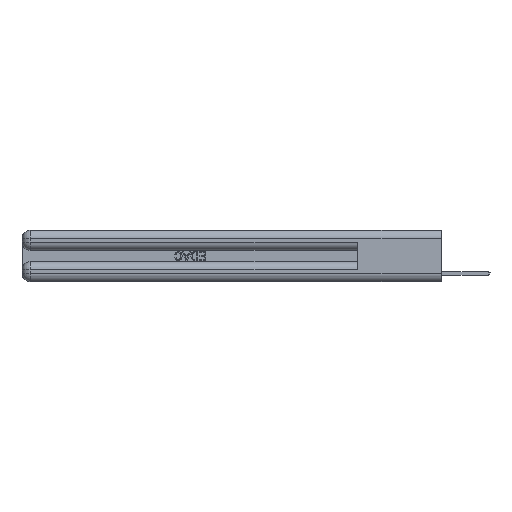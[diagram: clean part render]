
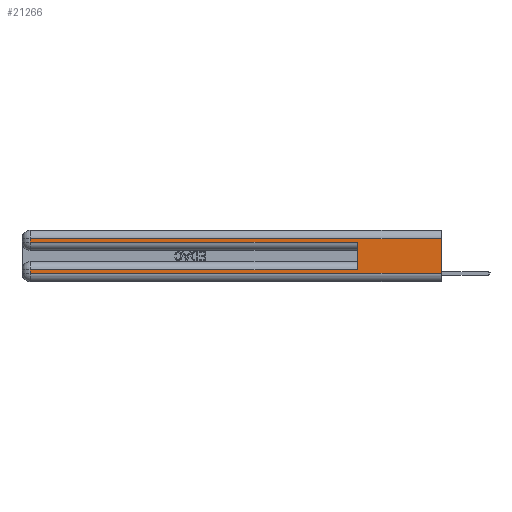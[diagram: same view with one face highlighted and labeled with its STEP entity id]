
A CAD part, left-side view. The second image highlights one B-rep face of the part: STEP entity #21266.
In plain terms, the highlighted planar face has unit normal (-1, 0, 0).
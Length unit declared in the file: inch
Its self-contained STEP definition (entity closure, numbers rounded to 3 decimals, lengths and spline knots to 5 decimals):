
#546 = DIRECTION ( 'NONE',  ( 1., 0., 0. ) ) ;
#887 = LINE ( 'NONE', #25383, #1001 ) ;
#1001 = VECTOR ( 'NONE', #10462, 39.37008 ) ;
#1051 = VECTOR ( 'NONE', #24910, 39.37008 ) ;
#1448 = AXIS2_PLACEMENT_3D ( 'NONE', #28660, #546, #10932 ) ;
#1958 = CARTESIAN_POINT ( 'NONE',  ( 0., 2.94, 0.06 ) ) ;
#3418 = CARTESIAN_POINT ( 'NONE',  ( 0., 0., 0.31 ) ) ;
#3622 = CARTESIAN_POINT ( 'NONE',  ( 0., 0.6, 0.085 ) ) ;
#4001 = DIRECTION ( 'NONE',  ( 0., -1., 0. ) ) ;
#4918 = VERTEX_POINT ( 'NONE', #3418 ) ;
#4954 = CARTESIAN_POINT ( 'NONE',  ( 0., 2.94, 0.31 ) ) ;
#4985 = CARTESIAN_POINT ( 'NONE',  ( 0., 2.94, 0.285 ) ) ;
#5174 = VERTEX_POINT ( 'NONE', #1958 ) ;
#5226 = EDGE_CURVE ( 'NONE', #13327, #26581, #20257, .T. ) ;
#5734 = LINE ( 'NONE', #5896, #10826 ) ;
#5896 = CARTESIAN_POINT ( 'NONE',  ( 0., 2.94, 0.37 ) ) ;
#7226 = ORIENTED_EDGE ( 'NONE', *, *, #17500, .T. ) ;
#7757 = VERTEX_POINT ( 'NONE', #12600 ) ;
#8492 = CARTESIAN_POINT ( 'NONE',  ( 0., 0.6, 0.285 ) ) ;
#9672 = LINE ( 'NONE', #22571, #1051 ) ;
#9835 = LINE ( 'NONE', #30186, #29101 ) ;
#9918 = VERTEX_POINT ( 'NONE', #8492 ) ;
#10306 = EDGE_CURVE ( 'NONE', #4918, #7757, #30637, .T. ) ;
#10462 = DIRECTION ( 'NONE',  ( 0., 0., 1. ) ) ;
#10665 = VECTOR ( 'NONE', #4001, 39.37008 ) ;
#10826 = VECTOR ( 'NONE', #20621, 39.37008 ) ;
#10932 = DIRECTION ( 'NONE',  ( 0., 0., -1. ) ) ;
#11837 = EDGE_CURVE ( 'NONE', #5174, #7757, #24356, .T. ) ;
#12512 = VECTOR ( 'NONE', #26177, 39.37008 ) ;
#12564 = ORIENTED_EDGE ( 'NONE', *, *, #10306, .F. ) ;
#12600 = CARTESIAN_POINT ( 'NONE',  ( 0., 0., 0.06 ) ) ;
#12888 = ORIENTED_EDGE ( 'NONE', *, *, #11837, .T. ) ;
#13202 = ORIENTED_EDGE ( 'NONE', *, *, #5226, .T. ) ;
#13327 = VERTEX_POINT ( 'NONE', #3622 ) ;
#13931 = EDGE_LOOP ( 'NONE', ( #12564, #22596, #7226, #15927, #15708, #13202, #24129, #12888 ) ) ;
#13957 = VECTOR ( 'NONE', #14703, 39.37008 ) ;
#14703 = DIRECTION ( 'NONE',  ( 0., -1., 0. ) ) ;
#15708 = ORIENTED_EDGE ( 'NONE', *, *, #23524, .F. ) ;
#15927 = ORIENTED_EDGE ( 'NONE', *, *, #18769, .T. ) ;
#16229 = CARTESIAN_POINT ( 'NONE',  ( 0., 0., 0.37 ) ) ;
#16570 = CARTESIAN_POINT ( 'NONE',  ( 0., 0., 0.06 ) ) ;
#17500 = EDGE_CURVE ( 'NONE', #18907, #27612, #5734, .T. ) ;
#18769 = EDGE_CURVE ( 'NONE', #27612, #9918, #22007, .T. ) ;
#18907 = VERTEX_POINT ( 'NONE', #4954 ) ;
#19912 = DIRECTION ( 'NONE',  ( 0., 1., 0. ) ) ;
#20200 = VECTOR ( 'NONE', #30690, 39.37008 ) ;
#20257 = LINE ( 'NONE', #27588, #20200 ) ;
#20621 = DIRECTION ( 'NONE',  ( 0., 0., -1. ) ) ;
#21266 = ADVANCED_FACE ( 'NONE', ( #31299 ), #25684, .F. ) ;
#22007 = LINE ( 'NONE', #32107, #13957 ) ;
#22571 = CARTESIAN_POINT ( 'NONE',  ( 0., 2.94, 0.37 ) ) ;
#22596 = ORIENTED_EDGE ( 'NONE', *, *, #27273, .T. ) ;
#23524 = EDGE_CURVE ( 'NONE', #13327, #9918, #887, .T. ) ;
#24129 = ORIENTED_EDGE ( 'NONE', *, *, #26157, .T. ) ;
#24356 = LINE ( 'NONE', #16570, #10665 ) ;
#24821 = CARTESIAN_POINT ( 'NONE',  ( 0., 2.94, 0.085 ) ) ;
#24910 = DIRECTION ( 'NONE',  ( 0., 0., -1. ) ) ;
#25383 = CARTESIAN_POINT ( 'NONE',  ( 0., 0.6, 0.145 ) ) ;
#25684 = PLANE ( 'NONE',  #1448 ) ;
#26157 = EDGE_CURVE ( 'NONE', #26581, #5174, #9672, .T. ) ;
#26177 = DIRECTION ( 'NONE',  ( 0., 0., -1. ) ) ;
#26581 = VERTEX_POINT ( 'NONE', #24821 ) ;
#27273 = EDGE_CURVE ( 'NONE', #4918, #18907, #9835, .T. ) ;
#27588 = CARTESIAN_POINT ( 'NONE',  ( 0., 0., 0.085 ) ) ;
#27612 = VERTEX_POINT ( 'NONE', #4985 ) ;
#28660 = CARTESIAN_POINT ( 'NONE',  ( 0., 0., 0.37 ) ) ;
#29101 = VECTOR ( 'NONE', #19912, 39.37008 ) ;
#30186 = CARTESIAN_POINT ( 'NONE',  ( 0., 0., 0.31 ) ) ;
#30637 = LINE ( 'NONE', #16229, #12512 ) ;
#30690 = DIRECTION ( 'NONE',  ( 0., 1., 0. ) ) ;
#31299 = FACE_OUTER_BOUND ( 'NONE', #13931, .T. ) ;
#32107 = CARTESIAN_POINT ( 'NONE',  ( 0., 0., 0.285 ) ) ;
